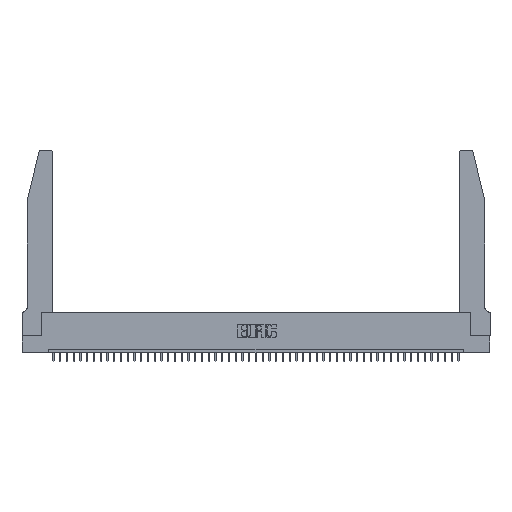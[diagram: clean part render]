
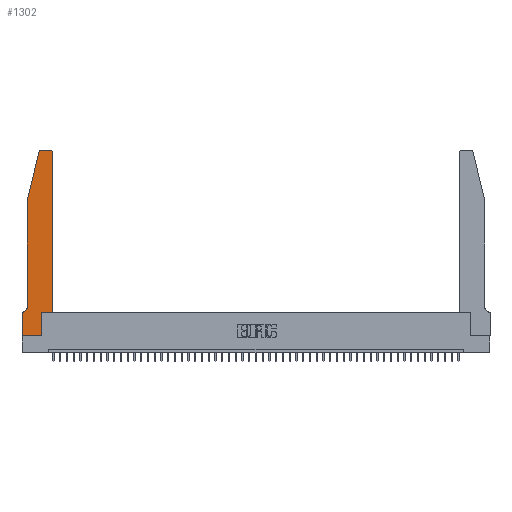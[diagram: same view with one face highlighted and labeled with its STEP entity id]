
A CAD part, top view. The second image highlights one B-rep face of the part: STEP entity #1302.
In plain terms, the highlighted planar face has unit normal (0, 0, 1).
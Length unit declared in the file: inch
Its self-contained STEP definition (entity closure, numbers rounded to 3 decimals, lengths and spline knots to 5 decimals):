
#171 = ORIENTED_EDGE ( 'NONE', *, *, #22971, .T. ) ;
#616 = EDGE_CURVE ( 'NONE', #19470, #46240, #31992, .T. ) ;
#657 = CARTESIAN_POINT ( 'NONE',  ( 0.0755, 2., 0.37 ) ) ;
#877 = CARTESIAN_POINT ( 'NONE',  ( 0.25487, 2.72718, 0.37 ) ) ;
#1249 = DIRECTION ( 'NONE',  ( 1., 0., 0. ) ) ;
#1302 = ADVANCED_FACE ( 'NONE', ( #31263 ), #11963, .T. ) ;
#1364 = DIRECTION ( 'NONE',  ( 1., 0., 0. ) ) ;
#1433 = CARTESIAN_POINT ( 'NONE',  ( 0.284, 2.72, 0.37 ) ) ;
#1952 = EDGE_CURVE ( 'NONE', #35510, #32408, #23781, .T. ) ;
#2889 = VECTOR ( 'NONE', #1364, 39.37008 ) ;
#4334 = VECTOR ( 'NONE', #16537, 39.37008 ) ;
#4500 = EDGE_CURVE ( 'NONE', #46240, #32625, #9631, .T. ) ;
#5999 = CARTESIAN_POINT ( 'NONE',  ( 0.2605, 2.75, 0.37 ) ) ;
#6406 = ORIENTED_EDGE ( 'NONE', *, *, #10258, .T. ) ;
#7320 = EDGE_CURVE ( 'NONE', #39531, #32947, #40088, .T. ) ;
#7487 = CARTESIAN_POINT ( 'NONE',  ( 0.2865, 0.35, 0.37 ) ) ;
#8353 = VERTEX_POINT ( 'NONE', #15398 ) ;
#8638 = VERTEX_POINT ( 'NONE', #21942 ) ;
#8997 = CARTESIAN_POINT ( 'NONE',  ( 0.4505, 0.35, 0.37 ) ) ;
#9603 = DIRECTION ( 'NONE',  ( -1., 0., 0. ) ) ;
#9631 = LINE ( 'NONE', #24524, #29020 ) ;
#9663 = EDGE_CURVE ( 'NONE', #8353, #8638, #44757, .T. ) ;
#10258 = EDGE_CURVE ( 'NONE', #42154, #32834, #23884, .T. ) ;
#10850 = LINE ( 'NONE', #5999, #36257 ) ;
#11052 = EDGE_CURVE ( 'NONE', #8638, #12663, #35524, .T. ) ;
#11750 = DIRECTION ( 'NONE',  ( 0., 0., -1. ) ) ;
#11782 = CARTESIAN_POINT ( 'NONE',  ( 0.4505, 2.72, 0.37 ) ) ;
#11963 = PLANE ( 'NONE',  #42816 ) ;
#12002 = CARTESIAN_POINT ( 'NONE',  ( 0.2865, 0.35, 0.37 ) ) ;
#12663 = VERTEX_POINT ( 'NONE', #41878 ) ;
#13492 = CARTESIAN_POINT ( 'NONE',  ( 0., 0., 0.37 ) ) ;
#13997 = AXIS2_PLACEMENT_3D ( 'NONE', #1433, #41688, #45534 ) ;
#14583 = CARTESIAN_POINT ( 'NONE',  ( 0.4505, 0.35, 0.37 ) ) ;
#15398 = CARTESIAN_POINT ( 'NONE',  ( 0.0755, 0.42, 0.37 ) ) ;
#15985 = LINE ( 'NONE', #34838, #43970 ) ;
#16460 = DIRECTION ( 'NONE',  ( 1., 0., 0. ) ) ;
#16537 = DIRECTION ( 'NONE',  ( 1., 0., 0. ) ) ;
#16574 = CARTESIAN_POINT ( 'NONE',  ( 0., 0.35, 0.37 ) ) ;
#16720 = ORIENTED_EDGE ( 'NONE', *, *, #23404, .T. ) ;
#17386 = LINE ( 'NONE', #43509, #41641 ) ;
#17756 = LINE ( 'NONE', #14583, #34112 ) ;
#18766 = CARTESIAN_POINT ( 'NONE',  ( 0.284, 2.75, 0.37 ) ) ;
#19405 = CARTESIAN_POINT ( 'NONE',  ( 0.4205, 2.72, 0.37 ) ) ;
#19470 = VERTEX_POINT ( 'NONE', #18766 ) ;
#20343 = DIRECTION ( 'NONE',  ( 0., -1., 0. ) ) ;
#20918 = ORIENTED_EDGE ( 'NONE', *, *, #32853, .T. ) ;
#21942 = CARTESIAN_POINT ( 'NONE',  ( 0.0055, 0.35, 0.37 ) ) ;
#22189 = AXIS2_PLACEMENT_3D ( 'NONE', #34724, #11750, #41301 ) ;
#22751 = LINE ( 'NONE', #12002, #45736 ) ;
#22971 = EDGE_CURVE ( 'NONE', #32834, #39531, #17756, .T. ) ;
#23404 = EDGE_CURVE ( 'NONE', #32408, #42154, #22751, .T. ) ;
#23781 = LINE ( 'NONE', #42109, #2889 ) ;
#23870 = VECTOR ( 'NONE', #9603, 39.37008 ) ;
#23884 = LINE ( 'NONE', #8997, #4334 ) ;
#24524 = CARTESIAN_POINT ( 'NONE',  ( 0.0755, 2., 0.37 ) ) ;
#25027 = DIRECTION ( 'NONE',  ( -1., 0., 0. ) ) ;
#26304 = ORIENTED_EDGE ( 'NONE', *, *, #616, .T. ) ;
#27035 = ORIENTED_EDGE ( 'NONE', *, *, #7320, .T. ) ;
#27260 = DIRECTION ( 'NONE',  ( 0., -1., 0. ) ) ;
#27381 = CARTESIAN_POINT ( 'NONE',  ( 0.2865, 0., 0.37 ) ) ;
#28932 = CARTESIAN_POINT ( 'NONE',  ( 0.4205, 2.75, 0.37 ) ) ;
#29020 = VECTOR ( 'NONE', #46689, 39.37008 ) ;
#30656 = DIRECTION ( 'NONE',  ( 0., 0., 1. ) ) ;
#31263 = FACE_OUTER_BOUND ( 'NONE', #38160, .T. ) ;
#31349 = CARTESIAN_POINT ( 'NONE',  ( 0.0755, 0.35, 0.37 ) ) ;
#31900 = ORIENTED_EDGE ( 'NONE', *, *, #44935, .T. ) ;
#31992 = CIRCLE ( 'NONE', #13997, 0.03 ) ;
#32408 = VERTEX_POINT ( 'NONE', #27381 ) ;
#32625 = VERTEX_POINT ( 'NONE', #657 ) ;
#32834 = VERTEX_POINT ( 'NONE', #34595 ) ;
#32853 = EDGE_CURVE ( 'NONE', #32625, #8353, #15985, .T. ) ;
#32947 = VERTEX_POINT ( 'NONE', #28932 ) ;
#32993 = EDGE_CURVE ( 'NONE', #32947, #19470, #10850, .T. ) ;
#33122 = AXIS2_PLACEMENT_3D ( 'NONE', #19405, #30656, #16460 ) ;
#33794 = ORIENTED_EDGE ( 'NONE', *, *, #11052, .T. ) ;
#34021 = DIRECTION ( 'NONE',  ( 0., 1., 0. ) ) ;
#34112 = VECTOR ( 'NONE', #40239, 39.37008 ) ;
#34595 = CARTESIAN_POINT ( 'NONE',  ( 0.4505, 0.35, 0.37 ) ) ;
#34724 = CARTESIAN_POINT ( 'NONE',  ( 0.0055, 0.42, 0.37 ) ) ;
#34838 = CARTESIAN_POINT ( 'NONE',  ( 0.0755, 2., 0.37 ) ) ;
#35510 = VERTEX_POINT ( 'NONE', #13492 ) ;
#35524 = LINE ( 'NONE', #31349, #23870 ) ;
#36257 = VECTOR ( 'NONE', #25027, 39.37008 ) ;
#36352 = ORIENTED_EDGE ( 'NONE', *, *, #9663, .T. ) ;
#38126 = DIRECTION ( 'NONE',  ( 0., 0., 1. ) ) ;
#38160 = EDGE_LOOP ( 'NONE', ( #39543, #26304, #47816, #20918, #36352, #33794, #31900, #39026, #16720, #6406, #171, #27035 ) ) ;
#39026 = ORIENTED_EDGE ( 'NONE', *, *, #1952, .T. ) ;
#39531 = VERTEX_POINT ( 'NONE', #11782 ) ;
#39543 = ORIENTED_EDGE ( 'NONE', *, *, #32993, .T. ) ;
#40088 = CIRCLE ( 'NONE', #33122, 0.03 ) ;
#40239 = DIRECTION ( 'NONE',  ( 0., 1., 0. ) ) ;
#41301 = DIRECTION ( 'NONE',  ( -1., 0., 0. ) ) ;
#41641 = VECTOR ( 'NONE', #20343, 39.37008 ) ;
#41688 = DIRECTION ( 'NONE',  ( 0., 0., 1. ) ) ;
#41878 = CARTESIAN_POINT ( 'NONE',  ( 0., 0.35, 0.37 ) ) ;
#42109 = CARTESIAN_POINT ( 'NONE',  ( 0., 0., 0.37 ) ) ;
#42154 = VERTEX_POINT ( 'NONE', #7487 ) ;
#42816 = AXIS2_PLACEMENT_3D ( 'NONE', #16574, #38126, #1249 ) ;
#43509 = CARTESIAN_POINT ( 'NONE',  ( 0., 0., 0.37 ) ) ;
#43970 = VECTOR ( 'NONE', #27260, 39.37008 ) ;
#44757 = CIRCLE ( 'NONE', #22189, 0.07 ) ;
#44935 = EDGE_CURVE ( 'NONE', #12663, #35510, #17386, .T. ) ;
#45534 = DIRECTION ( 'NONE',  ( 1., 0., 0. ) ) ;
#45736 = VECTOR ( 'NONE', #34021, 39.37008 ) ;
#46240 = VERTEX_POINT ( 'NONE', #877 ) ;
#46689 = DIRECTION ( 'NONE',  ( -0.239, -0.971, 0. ) ) ;
#47816 = ORIENTED_EDGE ( 'NONE', *, *, #4500, .T. ) ;
